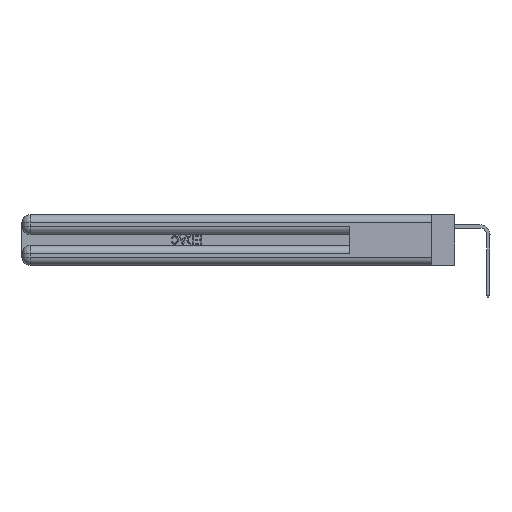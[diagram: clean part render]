
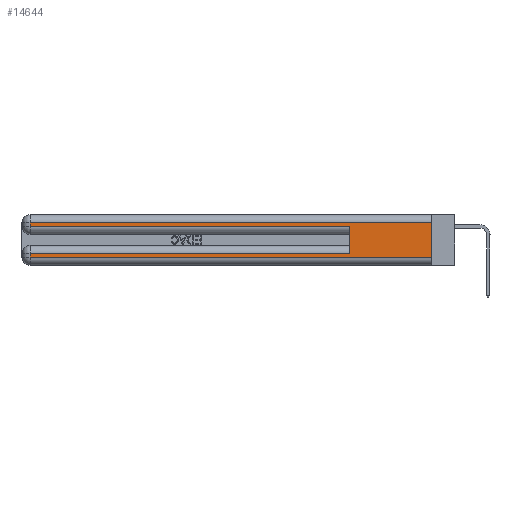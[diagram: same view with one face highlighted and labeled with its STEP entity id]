
A CAD part, left-side view. The second image highlights one B-rep face of the part: STEP entity #14644.
In plain terms, the highlighted planar face has unit normal (-1, 0, 0).
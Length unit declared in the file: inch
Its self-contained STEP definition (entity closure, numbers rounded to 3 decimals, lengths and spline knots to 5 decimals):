
#399 = LINE ( 'NONE', #15988, #33553 ) ;
#723 = VECTOR ( 'NONE', #25492, 39.37008 ) ;
#1073 = CARTESIAN_POINT ( 'NONE',  ( 0., 0.6, 0.145 ) ) ;
#1488 = VECTOR ( 'NONE', #22670, 39.37008 ) ;
#2429 = FACE_OUTER_BOUND ( 'NONE', #39364, .T. ) ;
#2956 = EDGE_CURVE ( 'NONE', #27438, #36929, #27310, .T. ) ;
#4732 = ORIENTED_EDGE ( 'NONE', *, *, #6452, .T. ) ;
#4762 = EDGE_CURVE ( 'NONE', #21855, #16004, #35549, .T. ) ;
#5216 = PLANE ( 'NONE',  #39762 ) ;
#5258 = EDGE_CURVE ( 'NONE', #27438, #11748, #399, .T. ) ;
#6267 = DIRECTION ( 'NONE',  ( 0., 1., 0. ) ) ;
#6452 = EDGE_CURVE ( 'NONE', #11748, #39810, #33828, .T. ) ;
#6501 = ORIENTED_EDGE ( 'NONE', *, *, #17136, .T. ) ;
#7427 = VERTEX_POINT ( 'NONE', #17958 ) ;
#7882 = DIRECTION ( 'NONE',  ( 0., -1., 0. ) ) ;
#8546 = EDGE_CURVE ( 'NONE', #21855, #7427, #34147, .T. ) ;
#8721 = VECTOR ( 'NONE', #26707, 39.37008 ) ;
#9948 = VECTOR ( 'NONE', #29877, 39.37008 ) ;
#10584 = CARTESIAN_POINT ( 'NONE',  ( 0., 0., 0.285 ) ) ;
#11533 = EDGE_CURVE ( 'NONE', #36502, #36929, #16591, .T. ) ;
#11668 = CARTESIAN_POINT ( 'NONE',  ( 0., 0., 0.37 ) ) ;
#11748 = VERTEX_POINT ( 'NONE', #28165 ) ;
#11799 = DIRECTION ( 'NONE',  ( 0., 0., -1. ) ) ;
#14644 = ADVANCED_FACE ( 'NONE', ( #2429 ), #5216, .F. ) ;
#15577 = VECTOR ( 'NONE', #7882, 39.37008 ) ;
#15988 = CARTESIAN_POINT ( 'NONE',  ( 0., 0., 0.31 ) ) ;
#16004 = VERTEX_POINT ( 'NONE', #30378 ) ;
#16128 = ORIENTED_EDGE ( 'NONE', *, *, #8546, .F. ) ;
#16591 = LINE ( 'NONE', #17714, #15577 ) ;
#17136 = EDGE_CURVE ( 'NONE', #16004, #36502, #26953, .T. ) ;
#17714 = CARTESIAN_POINT ( 'NONE',  ( 0., 0., 0.06 ) ) ;
#17958 = CARTESIAN_POINT ( 'NONE',  ( 0., 0.6, 0.285 ) ) ;
#19051 = CARTESIAN_POINT ( 'NONE',  ( 0., 0., 0.31 ) ) ;
#19258 = CARTESIAN_POINT ( 'NONE',  ( 0., 2.94, 0.37 ) ) ;
#19804 = DIRECTION ( 'NONE',  ( 0., 0., -1. ) ) ;
#21664 = LINE ( 'NONE', #10584, #38431 ) ;
#21855 = VERTEX_POINT ( 'NONE', #23725 ) ;
#22670 = DIRECTION ( 'NONE',  ( 0., 1., 0. ) ) ;
#23009 = EDGE_CURVE ( 'NONE', #39810, #7427, #21664, .T. ) ;
#23725 = CARTESIAN_POINT ( 'NONE',  ( 0., 0.6, 0.085 ) ) ;
#25492 = DIRECTION ( 'NONE',  ( 0., 0., -1. ) ) ;
#25691 = ORIENTED_EDGE ( 'NONE', *, *, #11533, .T. ) ;
#26332 = VECTOR ( 'NONE', #19804, 39.37008 ) ;
#26577 = CARTESIAN_POINT ( 'NONE',  ( 0., 2.94, 0.37 ) ) ;
#26707 = DIRECTION ( 'NONE',  ( 0., 0., 1. ) ) ;
#26953 = LINE ( 'NONE', #26577, #9948 ) ;
#27110 = ORIENTED_EDGE ( 'NONE', *, *, #23009, .T. ) ;
#27310 = LINE ( 'NONE', #29195, #26332 ) ;
#27438 = VERTEX_POINT ( 'NONE', #19051 ) ;
#28165 = CARTESIAN_POINT ( 'NONE',  ( 0., 2.94, 0.31 ) ) ;
#29195 = CARTESIAN_POINT ( 'NONE',  ( 0., 0., 0.37 ) ) ;
#29703 = DIRECTION ( 'NONE',  ( 0., -1., 0. ) ) ;
#29877 = DIRECTION ( 'NONE',  ( 0., 0., -1. ) ) ;
#30104 = CARTESIAN_POINT ( 'NONE',  ( 0., 2.94, 0.06 ) ) ;
#30378 = CARTESIAN_POINT ( 'NONE',  ( 0., 2.94, 0.085 ) ) ;
#30862 = DIRECTION ( 'NONE',  ( 1., 0., 0. ) ) ;
#33429 = ORIENTED_EDGE ( 'NONE', *, *, #2956, .F. ) ;
#33553 = VECTOR ( 'NONE', #6267, 39.37008 ) ;
#33828 = LINE ( 'NONE', #19258, #723 ) ;
#34147 = LINE ( 'NONE', #1073, #8721 ) ;
#35233 = CARTESIAN_POINT ( 'NONE',  ( 0., 0., 0.085 ) ) ;
#35549 = LINE ( 'NONE', #35233, #1488 ) ;
#36350 = CARTESIAN_POINT ( 'NONE',  ( 0., 2.94, 0.285 ) ) ;
#36502 = VERTEX_POINT ( 'NONE', #30104 ) ;
#36929 = VERTEX_POINT ( 'NONE', #41425 ) ;
#38431 = VECTOR ( 'NONE', #29703, 39.37008 ) ;
#38991 = ORIENTED_EDGE ( 'NONE', *, *, #4762, .T. ) ;
#39364 = EDGE_LOOP ( 'NONE', ( #33429, #41269, #4732, #27110, #16128, #38991, #6501, #25691 ) ) ;
#39762 = AXIS2_PLACEMENT_3D ( 'NONE', #11668, #30862, #11799 ) ;
#39810 = VERTEX_POINT ( 'NONE', #36350 ) ;
#41269 = ORIENTED_EDGE ( 'NONE', *, *, #5258, .T. ) ;
#41425 = CARTESIAN_POINT ( 'NONE',  ( 0., 0., 0.06 ) ) ;
